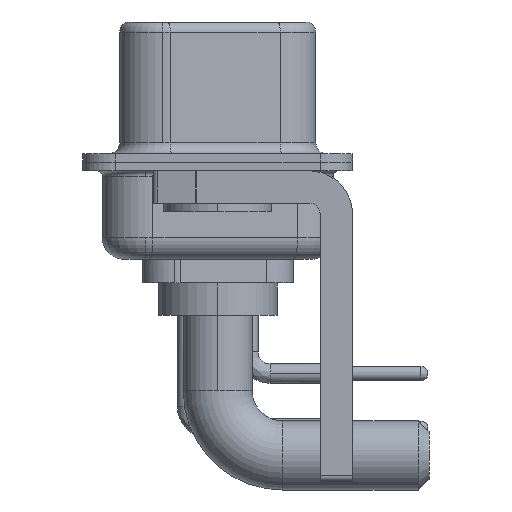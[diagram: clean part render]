
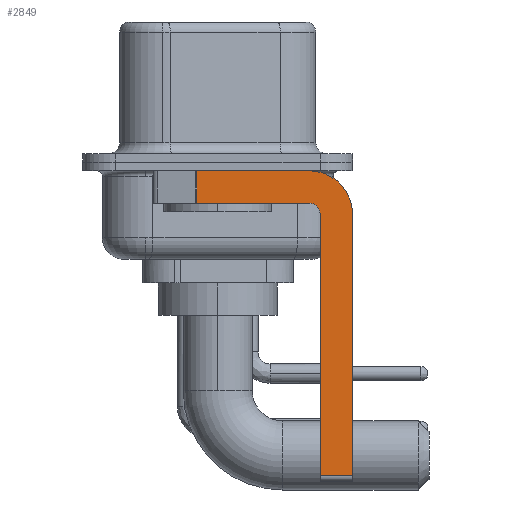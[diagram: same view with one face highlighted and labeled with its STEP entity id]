
A CAD part, left-side view. The second image highlights one B-rep face of the part: STEP entity #2849.
In plain terms, the highlighted planar face has unit normal (-1, 0, 0).
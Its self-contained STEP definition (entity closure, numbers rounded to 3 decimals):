
#264 = DIRECTION ( 'NONE',  ( 0., 0., -1. ) ) ;
#973 = VECTOR ( 'NONE', #3134, 1000. ) ;
#1386 = LINE ( 'NONE', #15583, #7208 ) ;
#1440 = VERTEX_POINT ( 'NONE', #6952 ) ;
#1558 = PLANE ( 'NONE',  #15414 ) ;
#2313 = DIRECTION ( 'NONE',  ( 1., 0., 0. ) ) ;
#2455 = AXIS2_PLACEMENT_3D ( 'NONE', #6808, #6459, #10220 ) ;
#2476 = CARTESIAN_POINT ( 'NONE',  ( -2.9, 0.978, -1.9 ) ) ;
#2849 = ADVANCED_FACE ( 'NONE', ( #12694 ), #1558, .F. ) ;
#2886 = LINE ( 'NONE', #18980, #14904 ) ;
#3134 = DIRECTION ( 'NONE',  ( 0., 0., -1. ) ) ;
#3155 = CARTESIAN_POINT ( 'NONE',  ( -2.9, -4.75, -14.55 ) ) ;
#3162 = ORIENTED_EDGE ( 'NONE', *, *, #5524, .T. ) ;
#4329 = EDGE_CURVE ( 'NONE', #9387, #17911, #1386, .T. ) ;
#4620 = ORIENTED_EDGE ( 'NONE', *, *, #7913, .F. ) ;
#4695 = VECTOR ( 'NONE', #9779, 1000. ) ;
#4885 = DIRECTION ( 'NONE',  ( 0., 0., 1. ) ) ;
#5374 = CARTESIAN_POINT ( 'NONE',  ( -2.9, -4.25, -1.9 ) ) ;
#5524 = EDGE_CURVE ( 'NONE', #20348, #17911, #18700, .T. ) ;
#5635 = VERTEX_POINT ( 'NONE', #17279 ) ;
#6459 = DIRECTION ( 'NONE',  ( -1., 0., 0. ) ) ;
#6674 = LINE ( 'NONE', #5374, #23131 ) ;
#6808 = CARTESIAN_POINT ( 'NONE',  ( -2.9, -4.25, -2.4 ) ) ;
#6943 = ORIENTED_EDGE ( 'NONE', *, *, #20740, .F. ) ;
#6952 = CARTESIAN_POINT ( 'NONE',  ( -2.9, 0.978, -0.4 ) ) ;
#7208 = VECTOR ( 'NONE', #16040, 1000. ) ;
#7390 = VERTEX_POINT ( 'NONE', #12561 ) ;
#7562 = ORIENTED_EDGE ( 'NONE', *, *, #18486, .F. ) ;
#7913 = EDGE_CURVE ( 'NONE', #7390, #16436, #6674, .T. ) ;
#9387 = VERTEX_POINT ( 'NONE', #11183 ) ;
#9677 = EDGE_CURVE ( 'NONE', #1440, #5635, #14210, .T. ) ;
#9779 = DIRECTION ( 'NONE',  ( 0., -1., 0. ) ) ;
#10009 = EDGE_CURVE ( 'NONE', #1440, #16436, #18422, .T. ) ;
#10220 = DIRECTION ( 'NONE',  ( 0., 0., 1. ) ) ;
#10233 = CARTESIAN_POINT ( 'NONE',  ( -2.9, 3., -0.4 ) ) ;
#10727 = CARTESIAN_POINT ( 'NONE',  ( -2.9, -4.25, -2.4 ) ) ;
#11183 = CARTESIAN_POINT ( 'NONE',  ( -2.9, -6.25, -2.4 ) ) ;
#11477 = CARTESIAN_POINT ( 'NONE',  ( -2.9, -4.25, -2.4 ) ) ;
#11740 = VECTOR ( 'NONE', #21030, 1000. ) ;
#11889 = AXIS2_PLACEMENT_3D ( 'NONE', #11477, #2313, #20161 ) ;
#12085 = DIRECTION ( 'NONE',  ( 0., 1., 0. ) ) ;
#12561 = CARTESIAN_POINT ( 'NONE',  ( -2.9, -4.25, -1.9 ) ) ;
#12694 = FACE_OUTER_BOUND ( 'NONE', #20942, .T. ) ;
#12763 = VERTEX_POINT ( 'NONE', #16422 ) ;
#13070 = ORIENTED_EDGE ( 'NONE', *, *, #4329, .F. ) ;
#13146 = ORIENTED_EDGE ( 'NONE', *, *, #20543, .F. ) ;
#14210 = LINE ( 'NONE', #10233, #11740 ) ;
#14817 = CIRCLE ( 'NONE', #2455, 0.5 ) ;
#14904 = VECTOR ( 'NONE', #4885, 1000. ) ;
#15295 = CARTESIAN_POINT ( 'NONE',  ( -2.9, -4.25, -14.55 ) ) ;
#15414 = AXIS2_PLACEMENT_3D ( 'NONE', #10727, #17752, #264 ) ;
#15583 = CARTESIAN_POINT ( 'NONE',  ( -2.9, -6.25, -2.4 ) ) ;
#16040 = DIRECTION ( 'NONE',  ( 0., 0., -1. ) ) ;
#16373 = CIRCLE ( 'NONE', #11889, 2. ) ;
#16422 = CARTESIAN_POINT ( 'NONE',  ( -2.9, -4.75, -2.4 ) ) ;
#16436 = VERTEX_POINT ( 'NONE', #19811 ) ;
#17279 = CARTESIAN_POINT ( 'NONE',  ( -2.9, -4.25, -0.4 ) ) ;
#17752 = DIRECTION ( 'NONE',  ( 1., 0., 0. ) ) ;
#17911 = VERTEX_POINT ( 'NONE', #18819 ) ;
#18287 = ORIENTED_EDGE ( 'NONE', *, *, #9677, .F. ) ;
#18422 = LINE ( 'NONE', #2476, #973 ) ;
#18486 = EDGE_CURVE ( 'NONE', #12763, #7390, #14817, .T. ) ;
#18700 = LINE ( 'NONE', #15295, #4695 ) ;
#18819 = CARTESIAN_POINT ( 'NONE',  ( -2.9, -6.25, -14.55 ) ) ;
#18980 = CARTESIAN_POINT ( 'NONE',  ( -2.9, -4.75, -14.8 ) ) ;
#19811 = CARTESIAN_POINT ( 'NONE',  ( -2.9, 0.978, -1.9 ) ) ;
#20161 = DIRECTION ( 'NONE',  ( 0., 0., -1. ) ) ;
#20348 = VERTEX_POINT ( 'NONE', #3155 ) ;
#20543 = EDGE_CURVE ( 'NONE', #5635, #9387, #16373, .T. ) ;
#20740 = EDGE_CURVE ( 'NONE', #20348, #12763, #2886, .T. ) ;
#20942 = EDGE_LOOP ( 'NONE', ( #18287, #21326, #4620, #7562, #6943, #3162, #13070, #13146 ) ) ;
#21030 = DIRECTION ( 'NONE',  ( 0., -1., 0. ) ) ;
#21326 = ORIENTED_EDGE ( 'NONE', *, *, #10009, .T. ) ;
#23131 = VECTOR ( 'NONE', #12085, 1000. ) ;
